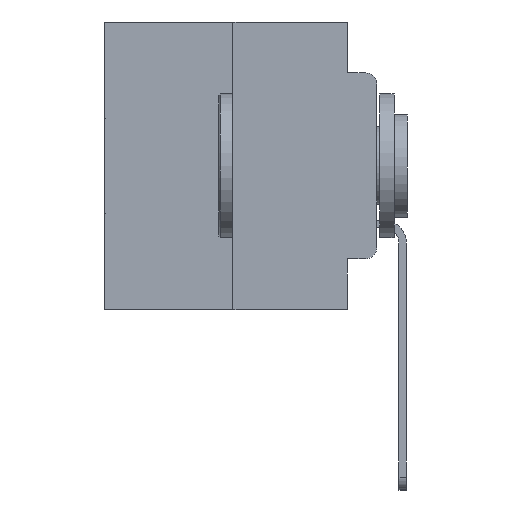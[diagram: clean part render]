
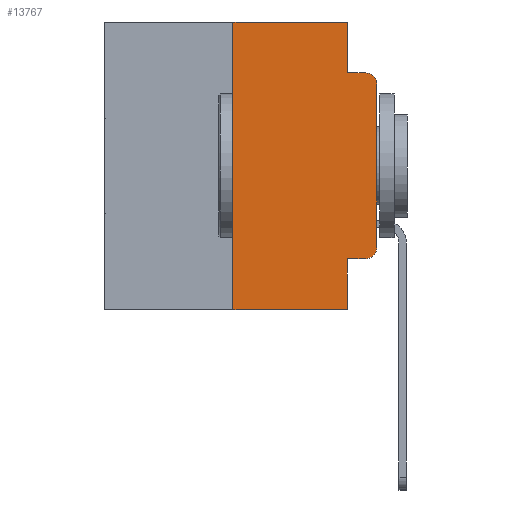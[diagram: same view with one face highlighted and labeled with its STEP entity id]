
A CAD part, left-side view. The second image highlights one B-rep face of the part: STEP entity #13767.
In plain terms, the highlighted planar face has unit normal (-1, 0, 0).
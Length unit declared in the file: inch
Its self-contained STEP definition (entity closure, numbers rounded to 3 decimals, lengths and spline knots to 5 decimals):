
#47 = CIRCLE ( 'NONE', #20211, 0.02 ) ;
#460 = DIRECTION ( 'NONE',  ( -1., 0., 0. ) ) ;
#685 = DIRECTION ( 'NONE',  ( 0., -1., 0. ) ) ;
#897 = DIRECTION ( 'NONE',  ( 1., 0., 0. ) ) ;
#977 = EDGE_CURVE ( 'NONE', #3975, #1344, #16186, .T. ) ;
#1035 = CARTESIAN_POINT ( 'NONE',  ( 0., 0.473, -0.5 ) ) ;
#1344 = VERTEX_POINT ( 'NONE', #19347 ) ;
#1858 = CARTESIAN_POINT ( 'NONE',  ( 0., 0., 0. ) ) ;
#1976 = DIRECTION ( 'NONE',  ( 0., 0., 1. ) ) ;
#2212 = AXIS2_PLACEMENT_3D ( 'NONE', #17863, #3971, #20152 ) ;
#2290 = ORIENTED_EDGE ( 'NONE', *, *, #8123, .F. ) ;
#2308 = VECTOR ( 'NONE', #13647, 39.37008 ) ;
#3076 = ORIENTED_EDGE ( 'NONE', *, *, #11344, .F. ) ;
#3669 = VECTOR ( 'NONE', #18969, 39.37008 ) ;
#3778 = VECTOR ( 'NONE', #18158, 39.37008 ) ;
#3971 = DIRECTION ( 'NONE',  ( -1., 0., 0. ) ) ;
#3975 = VERTEX_POINT ( 'NONE', #5138 ) ;
#4060 = FACE_OUTER_BOUND ( 'NONE', #16852, .T. ) ;
#4994 = VERTEX_POINT ( 'NONE', #9078 ) ;
#5032 = VERTEX_POINT ( 'NONE', #16362 ) ;
#5138 = CARTESIAN_POINT ( 'NONE',  ( 0., 0., -0.3915 ) ) ;
#5246 = ORIENTED_EDGE ( 'NONE', *, *, #977, .T. ) ;
#5407 = DIRECTION ( 'NONE',  ( 0., 0., -1. ) ) ;
#5549 = VERTEX_POINT ( 'NONE', #6476 ) ;
#6034 = CARTESIAN_POINT ( 'NONE',  ( 0., 0.02, -0.4115 ) ) ;
#6205 = VERTEX_POINT ( 'NONE', #15703 ) ;
#6476 = CARTESIAN_POINT ( 'NONE',  ( 0., 0.25, 0. ) ) ;
#6505 = LINE ( 'NONE', #19263, #24046 ) ;
#6734 = ORIENTED_EDGE ( 'NONE', *, *, #11668, .T. ) ;
#6800 = VECTOR ( 'NONE', #5407, 39.37008 ) ;
#8123 = EDGE_CURVE ( 'NONE', #6205, #11208, #13720, .T. ) ;
#9078 = CARTESIAN_POINT ( 'NONE',  ( 0., 0.051, -0.4115 ) ) ;
#9909 = VECTOR ( 'NONE', #21944, 39.37008 ) ;
#10066 = ORIENTED_EDGE ( 'NONE', *, *, #23173, .T. ) ;
#10323 = PLANE ( 'NONE',  #29443 ) ;
#11155 = ORIENTED_EDGE ( 'NONE', *, *, #12825, .T. ) ;
#11208 = VERTEX_POINT ( 'NONE', #22922 ) ;
#11317 = CARTESIAN_POINT ( 'NONE',  ( 0., 0.051, -0.4115 ) ) ;
#11344 = EDGE_CURVE ( 'NONE', #4994, #5032, #27042, .T. ) ;
#11668 = EDGE_CURVE ( 'NONE', #1344, #22574, #12526, .T. ) ;
#12526 = CIRCLE ( 'NONE', #2212, 0.02 ) ;
#12825 = EDGE_CURVE ( 'NONE', #22432, #5032, #24189, .T. ) ;
#13647 = DIRECTION ( 'NONE',  ( 0., -1., 0. ) ) ;
#13720 = LINE ( 'NONE', #16992, #6800 ) ;
#13767 = ADVANCED_FACE ( 'NONE', ( #4060 ), #10323, .F. ) ;
#14530 = CARTESIAN_POINT ( 'NONE',  ( 0., 0.02, -0.3915 ) ) ;
#15628 = EDGE_CURVE ( 'NONE', #5549, #6205, #6505, .T. ) ;
#15703 = CARTESIAN_POINT ( 'NONE',  ( 0., 0.051, 0. ) ) ;
#15873 = ORIENTED_EDGE ( 'NONE', *, *, #24487, .F. ) ;
#16031 = CARTESIAN_POINT ( 'NONE',  ( 0., 0.02, -0.0885 ) ) ;
#16084 = LINE ( 'NONE', #25621, #3669 ) ;
#16113 = CARTESIAN_POINT ( 'NONE',  ( 0., 0.25, 0. ) ) ;
#16186 = LINE ( 'NONE', #1858, #3778 ) ;
#16362 = CARTESIAN_POINT ( 'NONE',  ( 0., 0.051, -0.5 ) ) ;
#16841 = DIRECTION ( 'NONE',  ( 0., 0., -1. ) ) ;
#16852 = EDGE_LOOP ( 'NONE', ( #5246, #6734, #29112, #2290, #17618, #15873, #11155, #3076, #10066, #25717 ) ) ;
#16992 = CARTESIAN_POINT ( 'NONE',  ( 0., 0.051, 0. ) ) ;
#17278 = DIRECTION ( 'NONE',  ( 0., 0., -1. ) ) ;
#17618 = ORIENTED_EDGE ( 'NONE', *, *, #15628, .F. ) ;
#17863 = CARTESIAN_POINT ( 'NONE',  ( 0., 0.02, -0.1085 ) ) ;
#18158 = DIRECTION ( 'NONE',  ( 0., 0., 1. ) ) ;
#18321 = VERTEX_POINT ( 'NONE', #6034 ) ;
#18969 = DIRECTION ( 'NONE',  ( 0., -1., 0. ) ) ;
#19263 = CARTESIAN_POINT ( 'NONE',  ( 0., 0.473, 0. ) ) ;
#19347 = CARTESIAN_POINT ( 'NONE',  ( 0., 0., -0.1085 ) ) ;
#19464 = CARTESIAN_POINT ( 'NONE',  ( 0., 0.473, 0. ) ) ;
#20152 = DIRECTION ( 'NONE',  ( 0., 0., -1. ) ) ;
#20211 = AXIS2_PLACEMENT_3D ( 'NONE', #14530, #460, #16841 ) ;
#20750 = VECTOR ( 'NONE', #1976, 39.37008 ) ;
#21140 = VECTOR ( 'NONE', #25627, 39.37008 ) ;
#21407 = EDGE_CURVE ( 'NONE', #11208, #22574, #16084, .T. ) ;
#21944 = DIRECTION ( 'NONE',  ( 0., -1., 0. ) ) ;
#22432 = VERTEX_POINT ( 'NONE', #28789 ) ;
#22574 = VERTEX_POINT ( 'NONE', #16031 ) ;
#22922 = CARTESIAN_POINT ( 'NONE',  ( 0., 0.051, -0.0885 ) ) ;
#23173 = EDGE_CURVE ( 'NONE', #4994, #18321, #26036, .T. ) ;
#23410 = CARTESIAN_POINT ( 'NONE',  ( 0., 0.051, 0. ) ) ;
#24046 = VECTOR ( 'NONE', #685, 39.37008 ) ;
#24189 = LINE ( 'NONE', #1035, #9909 ) ;
#24487 = EDGE_CURVE ( 'NONE', #22432, #5549, #25955, .T. ) ;
#25621 = CARTESIAN_POINT ( 'NONE',  ( 0., 0.051, -0.0885 ) ) ;
#25627 = DIRECTION ( 'NONE',  ( 0., 0., -1. ) ) ;
#25717 = ORIENTED_EDGE ( 'NONE', *, *, #28150, .T. ) ;
#25955 = LINE ( 'NONE', #16113, #20750 ) ;
#26036 = LINE ( 'NONE', #11317, #2308 ) ;
#27042 = LINE ( 'NONE', #23410, #21140 ) ;
#28150 = EDGE_CURVE ( 'NONE', #18321, #3975, #47, .T. ) ;
#28789 = CARTESIAN_POINT ( 'NONE',  ( 0., 0.25, -0.5 ) ) ;
#29112 = ORIENTED_EDGE ( 'NONE', *, *, #21407, .F. ) ;
#29443 = AXIS2_PLACEMENT_3D ( 'NONE', #19464, #897, #17278 ) ;
